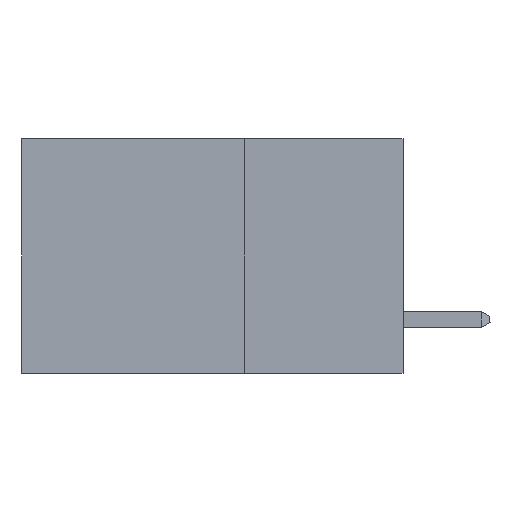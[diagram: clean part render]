
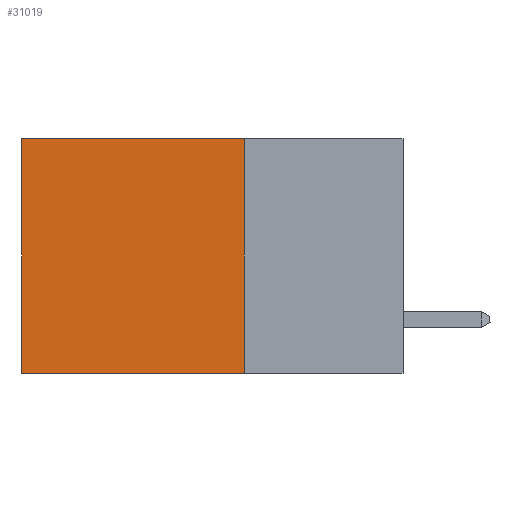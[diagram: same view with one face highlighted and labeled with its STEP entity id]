
A CAD part, left-side view. The second image highlights one B-rep face of the part: STEP entity #31019.
In plain terms, the highlighted planar face has unit normal (-1, 0, 0).
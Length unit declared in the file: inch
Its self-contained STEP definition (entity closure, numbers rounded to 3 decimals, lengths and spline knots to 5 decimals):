
#2103 = DIRECTION ( 'NONE',  ( 0., 1., 0. ) ) ;
#2997 = CARTESIAN_POINT ( 'NONE',  ( 0.2875, 0.25, -0.37 ) ) ;
#6658 = CARTESIAN_POINT ( 'NONE',  ( 0.2875, 0.25, 0. ) ) ;
#7876 = AXIS2_PLACEMENT_3D ( 'NONE', #34928, #10948, #39806 ) ;
#9891 = VERTEX_POINT ( 'NONE', #20094 ) ;
#10687 = VECTOR ( 'NONE', #23387, 39.37008 ) ;
#10841 = ORIENTED_EDGE ( 'NONE', *, *, #14276, .F. ) ;
#10948 = DIRECTION ( 'NONE',  ( 1., 0., 0. ) ) ;
#12532 = VERTEX_POINT ( 'NONE', #14149 ) ;
#14149 = CARTESIAN_POINT ( 'NONE',  ( 0.2875, 0.6, 0. ) ) ;
#14276 = EDGE_CURVE ( 'NONE', #9891, #28731, #18080, .T. ) ;
#16565 = VECTOR ( 'NONE', #2103, 39.37008 ) ;
#18080 = LINE ( 'NONE', #6658, #10687 ) ;
#20094 = CARTESIAN_POINT ( 'NONE',  ( 0.2875, 0.25, 0. ) ) ;
#21415 = FACE_OUTER_BOUND ( 'NONE', #32645, .T. ) ;
#21668 = CARTESIAN_POINT ( 'NONE',  ( 0.2875, 0.25, -0.37 ) ) ;
#23387 = DIRECTION ( 'NONE',  ( 0., 0., -1. ) ) ;
#24798 = VECTOR ( 'NONE', #42459, 39.37008 ) ;
#25244 = EDGE_CURVE ( 'NONE', #9891, #12532, #35664, .T. ) ;
#25910 = VECTOR ( 'NONE', #26806, 39.37008 ) ;
#25921 = CARTESIAN_POINT ( 'NONE',  ( 0.2875, 0.25, 0. ) ) ;
#26299 = CARTESIAN_POINT ( 'NONE',  ( 0.2875, 0.6, -0.37 ) ) ;
#26806 = DIRECTION ( 'NONE',  ( 0., 1., 0. ) ) ;
#27955 = ORIENTED_EDGE ( 'NONE', *, *, #35381, .F. ) ;
#28116 = PLANE ( 'NONE',  #7876 ) ;
#28731 = VERTEX_POINT ( 'NONE', #21668 ) ;
#30014 = ORIENTED_EDGE ( 'NONE', *, *, #42373, .T. ) ;
#31019 = ADVANCED_FACE ( 'NONE', ( #21415 ), #28116, .F. ) ;
#31095 = VERTEX_POINT ( 'NONE', #26299 ) ;
#31896 = CARTESIAN_POINT ( 'NONE',  ( 0.2875, 0.6, 0. ) ) ;
#32645 = EDGE_LOOP ( 'NONE', ( #30014, #27955, #10841, #33508 ) ) ;
#33508 = ORIENTED_EDGE ( 'NONE', *, *, #25244, .T. ) ;
#34928 = CARTESIAN_POINT ( 'NONE',  ( 0.2875, 0.25, 0. ) ) ;
#35381 = EDGE_CURVE ( 'NONE', #28731, #31095, #40755, .T. ) ;
#35664 = LINE ( 'NONE', #25921, #16565 ) ;
#38592 = LINE ( 'NONE', #31896, #24798 ) ;
#39806 = DIRECTION ( 'NONE',  ( 0., 0., -1. ) ) ;
#40755 = LINE ( 'NONE', #2997, #25910 ) ;
#42373 = EDGE_CURVE ( 'NONE', #12532, #31095, #38592, .T. ) ;
#42459 = DIRECTION ( 'NONE',  ( 0., 0., -1. ) ) ;
